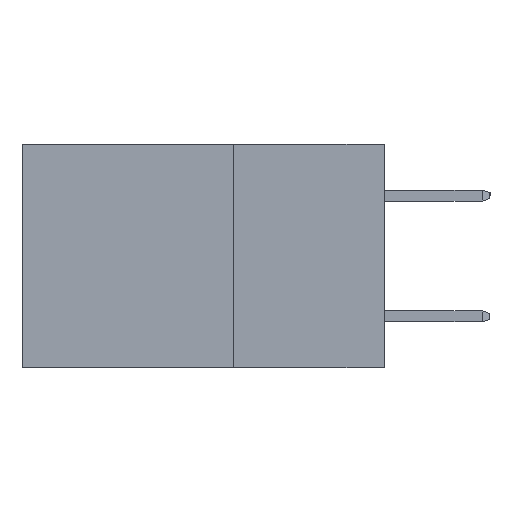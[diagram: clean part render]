
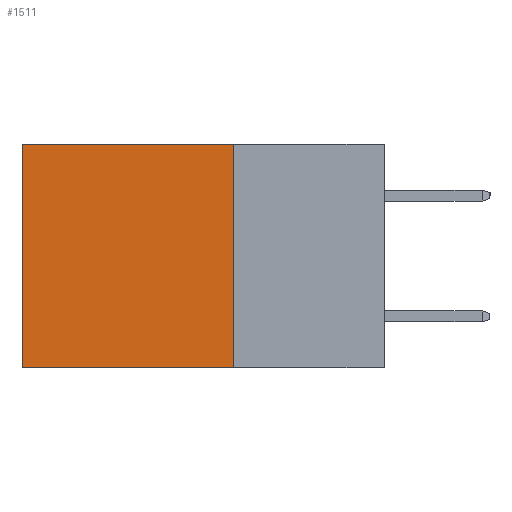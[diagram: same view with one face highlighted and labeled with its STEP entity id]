
A CAD part, left-side view. The second image highlights one B-rep face of the part: STEP entity #1511.
In plain terms, the highlighted planar face has unit normal (-1, 0, 0).
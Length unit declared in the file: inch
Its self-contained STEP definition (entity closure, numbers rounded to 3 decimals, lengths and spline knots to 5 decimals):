
#1347 = LINE ( 'NONE', #2272, #2602 ) ;
#1490 = EDGE_CURVE ( 'NONE', #4090, #2167, #1347, .T. ) ;
#1511 = ADVANCED_FACE ( 'NONE', ( #3079 ), #7037, .F. ) ;
#1624 = AXIS2_PLACEMENT_3D ( 'NONE', #2332, #6104, #10572 ) ;
#1820 = VECTOR ( 'NONE', #4365, 39.37008 ) ;
#2167 = VERTEX_POINT ( 'NONE', #5476 ) ;
#2272 = CARTESIAN_POINT ( 'NONE',  ( 0.2615, 0.25, 0. ) ) ;
#2332 = CARTESIAN_POINT ( 'NONE',  ( 0.2615, 0.25, -0.37 ) ) ;
#2383 = CARTESIAN_POINT ( 'NONE',  ( 0.2615, 0.25, -0.37 ) ) ;
#2602 = VECTOR ( 'NONE', #5000, 39.37008 ) ;
#2766 = VERTEX_POINT ( 'NONE', #11019 ) ;
#2957 = LINE ( 'NONE', #7899, #6786 ) ;
#3079 = FACE_OUTER_BOUND ( 'NONE', #12075, .T. ) ;
#4065 = LINE ( 'NONE', #8884, #6301 ) ;
#4075 = DIRECTION ( 'NONE',  ( 0., 0., -1. ) ) ;
#4090 = VERTEX_POINT ( 'NONE', #11649 ) ;
#4113 = EDGE_CURVE ( 'NONE', #4090, #12012, #10916, .T. ) ;
#4365 = DIRECTION ( 'NONE',  ( 0., 0., -1. ) ) ;
#5000 = DIRECTION ( 'NONE',  ( 0., 1., 0. ) ) ;
#5242 = ORIENTED_EDGE ( 'NONE', *, *, #6892, .T. ) ;
#5376 = CARTESIAN_POINT ( 'NONE',  ( 0.2615, 0.25, -0.37 ) ) ;
#5476 = CARTESIAN_POINT ( 'NONE',  ( 0.2615, 0.6, 0. ) ) ;
#6068 = ORIENTED_EDGE ( 'NONE', *, *, #8799, .F. ) ;
#6104 = DIRECTION ( 'NONE',  ( 1., 0., 0. ) ) ;
#6301 = VECTOR ( 'NONE', #8819, 39.37008 ) ;
#6786 = VECTOR ( 'NONE', #4075, 39.37008 ) ;
#6892 = EDGE_CURVE ( 'NONE', #2167, #2766, #2957, .T. ) ;
#7037 = PLANE ( 'NONE',  #1624 ) ;
#7899 = CARTESIAN_POINT ( 'NONE',  ( 0.2615, 0.6, -0.37 ) ) ;
#8112 = ORIENTED_EDGE ( 'NONE', *, *, #4113, .F. ) ;
#8799 = EDGE_CURVE ( 'NONE', #12012, #2766, #4065, .T. ) ;
#8819 = DIRECTION ( 'NONE',  ( 0., 1., 0. ) ) ;
#8884 = CARTESIAN_POINT ( 'NONE',  ( 0.2615, 0.25, -0.37 ) ) ;
#10572 = DIRECTION ( 'NONE',  ( 0., 0., -1. ) ) ;
#10875 = ORIENTED_EDGE ( 'NONE', *, *, #1490, .T. ) ;
#10916 = LINE ( 'NONE', #2383, #1820 ) ;
#11019 = CARTESIAN_POINT ( 'NONE',  ( 0.2615, 0.6, -0.37 ) ) ;
#11649 = CARTESIAN_POINT ( 'NONE',  ( 0.2615, 0.25, 0. ) ) ;
#12012 = VERTEX_POINT ( 'NONE', #5376 ) ;
#12075 = EDGE_LOOP ( 'NONE', ( #5242, #6068, #8112, #10875 ) ) ;
